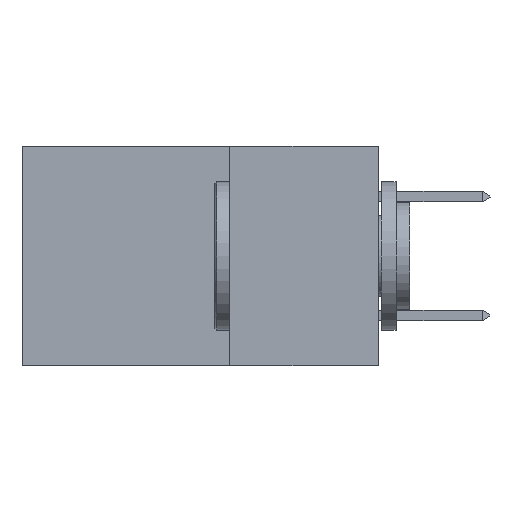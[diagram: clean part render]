
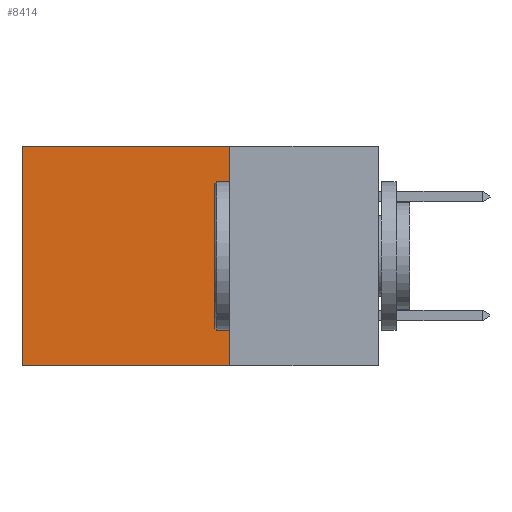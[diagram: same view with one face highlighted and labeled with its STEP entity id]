
A CAD part, left-side view. The second image highlights one B-rep face of the part: STEP entity #8414.
In plain terms, the highlighted planar face has unit normal (-1, 0, 0).
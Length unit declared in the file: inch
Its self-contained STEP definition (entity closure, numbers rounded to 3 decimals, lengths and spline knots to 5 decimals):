
#976 = CARTESIAN_POINT ( 'NONE',  ( 0.298, 0.25, 0. ) ) ;
#1345 = CARTESIAN_POINT ( 'NONE',  ( 0.298, 0.25, -0.37 ) ) ;
#1493 = DIRECTION ( 'NONE',  ( 1., 0., 0. ) ) ;
#3836 = CARTESIAN_POINT ( 'NONE',  ( 0.298, 0.25, -0.37 ) ) ;
#3877 = CARTESIAN_POINT ( 'NONE',  ( 0.298, 0.6, 0. ) ) ;
#4224 = EDGE_CURVE ( 'NONE', #13362, #28986, #11300, .T. ) ;
#4953 = VECTOR ( 'NONE', #19257, 39.37008 ) ;
#5003 = DIRECTION ( 'NONE',  ( 0., 0., -1. ) ) ;
#5053 = ORIENTED_EDGE ( 'NONE', *, *, #10580, .T. ) ;
#5867 = CARTESIAN_POINT ( 'NONE',  ( 0.298, 0.25, 0. ) ) ;
#7588 = ORIENTED_EDGE ( 'NONE', *, *, #10066, .F. ) ;
#8414 = ADVANCED_FACE ( 'NONE', ( #12530 ), #13334, .F. ) ;
#8618 = VECTOR ( 'NONE', #22510, 39.37008 ) ;
#10053 = VERTEX_POINT ( 'NONE', #976 ) ;
#10066 = EDGE_CURVE ( 'NONE', #10053, #13362, #26821, .T. ) ;
#10383 = LINE ( 'NONE', #21651, #28590 ) ;
#10580 = EDGE_CURVE ( 'NONE', #10053, #14564, #26051, .T. ) ;
#11300 = LINE ( 'NONE', #1345, #4953 ) ;
#12530 = FACE_OUTER_BOUND ( 'NONE', #17949, .T. ) ;
#13334 = PLANE ( 'NONE',  #28099 ) ;
#13362 = VERTEX_POINT ( 'NONE', #3836 ) ;
#14563 = DIRECTION ( 'NONE',  ( 0., 1., 0. ) ) ;
#14564 = VERTEX_POINT ( 'NONE', #3877 ) ;
#17949 = EDGE_LOOP ( 'NONE', ( #22381, #22529, #7588, #5053 ) ) ;
#18106 = DIRECTION ( 'NONE',  ( 0., 0., -1. ) ) ;
#19238 = CARTESIAN_POINT ( 'NONE',  ( 0.298, 0.25, 0. ) ) ;
#19257 = DIRECTION ( 'NONE',  ( 0., 1., 0. ) ) ;
#19686 = VECTOR ( 'NONE', #14563, 39.37008 ) ;
#20769 = CARTESIAN_POINT ( 'NONE',  ( 0.298, 0.6, -0.37 ) ) ;
#21651 = CARTESIAN_POINT ( 'NONE',  ( 0.298, 0.6, 0. ) ) ;
#22381 = ORIENTED_EDGE ( 'NONE', *, *, #27975, .T. ) ;
#22510 = DIRECTION ( 'NONE',  ( 0., 0., -1. ) ) ;
#22529 = ORIENTED_EDGE ( 'NONE', *, *, #4224, .F. ) ;
#26051 = LINE ( 'NONE', #19238, #19686 ) ;
#26821 = LINE ( 'NONE', #5867, #8618 ) ;
#27975 = EDGE_CURVE ( 'NONE', #14564, #28986, #10383, .T. ) ;
#28099 = AXIS2_PLACEMENT_3D ( 'NONE', #29948, #1493, #18106 ) ;
#28590 = VECTOR ( 'NONE', #5003, 39.37008 ) ;
#28986 = VERTEX_POINT ( 'NONE', #20769 ) ;
#29948 = CARTESIAN_POINT ( 'NONE',  ( 0.298, 0.25, 0. ) ) ;
